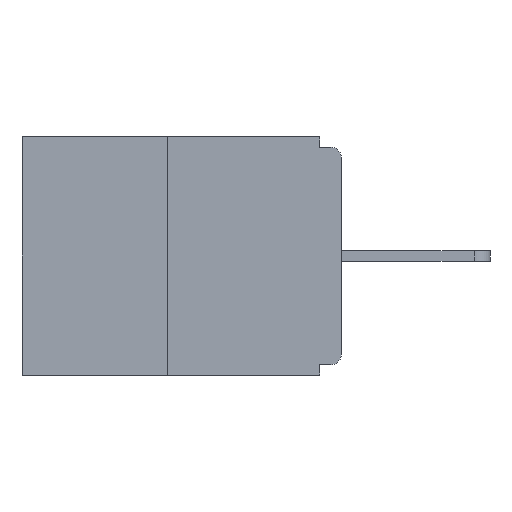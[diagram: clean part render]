
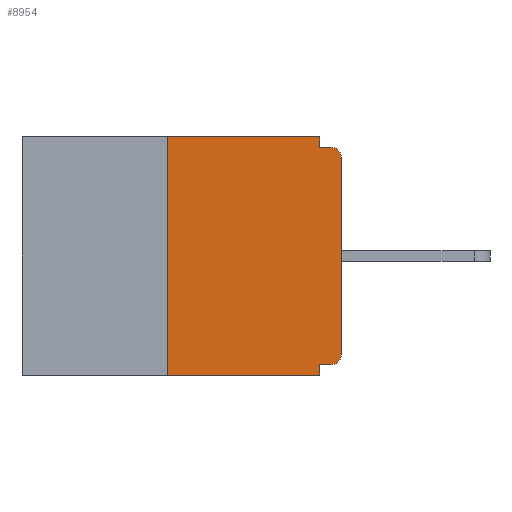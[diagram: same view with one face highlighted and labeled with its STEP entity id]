
A CAD part, left-side view. The second image highlights one B-rep face of the part: STEP entity #8954.
In plain terms, the highlighted planar face has unit normal (-1, 0, 0).
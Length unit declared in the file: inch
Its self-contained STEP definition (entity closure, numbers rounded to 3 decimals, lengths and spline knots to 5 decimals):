
#16 = CARTESIAN_POINT ( 'NONE',  ( 0., 0.015, -0.015 ) ) ;
#80 = VECTOR ( 'NONE', #10535, 39.37008 ) ;
#140 = ORIENTED_EDGE ( 'NONE', *, *, #8444, .F. ) ;
#161 = LINE ( 'NONE', #9205, #4442 ) ;
#212 = EDGE_CURVE ( 'NONE', #8233, #7573, #5155, .T. ) ;
#301 = VERTEX_POINT ( 'NONE', #8874 ) ;
#320 = ORIENTED_EDGE ( 'NONE', *, *, #418, .T. ) ;
#324 = CARTESIAN_POINT ( 'NONE',  ( 0., 0.46, 0. ) ) ;
#379 = DIRECTION ( 'NONE',  ( 0., 0., -1. ) ) ;
#418 = EDGE_CURVE ( 'NONE', #6286, #8233, #7456, .T. ) ;
#588 = DIRECTION ( 'NONE',  ( -1., 0., 0. ) ) ;
#603 = ORIENTED_EDGE ( 'NONE', *, *, #212, .T. ) ;
#849 = LINE ( 'NONE', #7314, #9579 ) ;
#899 = LINE ( 'NONE', #1636, #4601 ) ;
#989 = EDGE_CURVE ( 'NONE', #9513, #6377, #849, .T. ) ;
#1070 = FACE_OUTER_BOUND ( 'NONE', #1598, .T. ) ;
#1315 = VECTOR ( 'NONE', #6848, 39.37008 ) ;
#1461 = CARTESIAN_POINT ( 'NONE',  ( 0., 0., -0.328 ) ) ;
#1584 = CARTESIAN_POINT ( 'NONE',  ( 0., 0., -0.03 ) ) ;
#1594 = DIRECTION ( 'NONE',  ( 0., -1., 0. ) ) ;
#1598 = EDGE_LOOP ( 'NONE', ( #2621, #5974, #6229, #8746, #8062, #7811, #320, #603, #3981, #140 ) ) ;
#1636 = CARTESIAN_POINT ( 'NONE',  ( 0., 0.031, 0. ) ) ;
#1834 = LINE ( 'NONE', #324, #1315 ) ;
#2033 = AXIS2_PLACEMENT_3D ( 'NONE', #5449, #588, #6237 ) ;
#2140 = DIRECTION ( 'NONE',  ( 0., 0., -1. ) ) ;
#2203 = CARTESIAN_POINT ( 'NONE',  ( 0., 0.031, -0.343 ) ) ;
#2275 = LINE ( 'NONE', #1461, #5230 ) ;
#2278 = LINE ( 'NONE', #4780, #80 ) ;
#2409 = VERTEX_POINT ( 'NONE', #7207 ) ;
#2553 = CARTESIAN_POINT ( 'NONE',  ( 0., 0., 0. ) ) ;
#2621 = ORIENTED_EDGE ( 'NONE', *, *, #10112, .F. ) ;
#3011 = DIRECTION ( 'NONE',  ( -1., 0., 0. ) ) ;
#3078 = VERTEX_POINT ( 'NONE', #10090 ) ;
#3309 = CIRCLE ( 'NONE', #9323, 0.015 ) ;
#3534 = EDGE_CURVE ( 'NONE', #3078, #6286, #3309, .T. ) ;
#3981 = ORIENTED_EDGE ( 'NONE', *, *, #7483, .F. ) ;
#4133 = VECTOR ( 'NONE', #8020, 39.37008 ) ;
#4199 = DIRECTION ( 'NONE',  ( 0., 0., -1. ) ) ;
#4442 = VECTOR ( 'NONE', #5139, 39.37008 ) ;
#4601 = VECTOR ( 'NONE', #4199, 39.37008 ) ;
#4630 = EDGE_CURVE ( 'NONE', #3078, #9767, #2275, .T. ) ;
#4718 = CARTESIAN_POINT ( 'NONE',  ( 0., 0.031, -0.328 ) ) ;
#4780 = CARTESIAN_POINT ( 'NONE',  ( 0., 0., -0.015 ) ) ;
#5031 = PLANE ( 'NONE',  #5923 ) ;
#5133 = DIRECTION ( 'NONE',  ( 1., 0., 0. ) ) ;
#5139 = DIRECTION ( 'NONE',  ( 0., 0., 1. ) ) ;
#5155 = CIRCLE ( 'NONE', #2033, 0.015 ) ;
#5230 = VECTOR ( 'NONE', #7639, 39.37008 ) ;
#5240 = CARTESIAN_POINT ( 'NONE',  ( 0., 0., -0.313 ) ) ;
#5449 = CARTESIAN_POINT ( 'NONE',  ( 0., 0.015, -0.03 ) ) ;
#5496 = CARTESIAN_POINT ( 'NONE',  ( 0., 0.015, -0.313 ) ) ;
#5774 = CARTESIAN_POINT ( 'NONE',  ( 0., 0.46, 0. ) ) ;
#5923 = AXIS2_PLACEMENT_3D ( 'NONE', #5774, #5133, #10030 ) ;
#5929 = CARTESIAN_POINT ( 'NONE',  ( 0., 0.031, -0.343 ) ) ;
#5974 = ORIENTED_EDGE ( 'NONE', *, *, #10185, .F. ) ;
#6229 = ORIENTED_EDGE ( 'NONE', *, *, #989, .T. ) ;
#6237 = DIRECTION ( 'NONE',  ( 0., 0., -1. ) ) ;
#6286 = VERTEX_POINT ( 'NONE', #5240 ) ;
#6377 = VERTEX_POINT ( 'NONE', #5929 ) ;
#6848 = DIRECTION ( 'NONE',  ( 0., -1., 0. ) ) ;
#7207 = CARTESIAN_POINT ( 'NONE',  ( 0., 0.031, -0.015 ) ) ;
#7314 = CARTESIAN_POINT ( 'NONE',  ( 0., 0.46, -0.343 ) ) ;
#7449 = CARTESIAN_POINT ( 'NONE',  ( 0., 0.25, -0.343 ) ) ;
#7456 = LINE ( 'NONE', #2553, #4133 ) ;
#7483 = EDGE_CURVE ( 'NONE', #2409, #7573, #2278, .T. ) ;
#7573 = VERTEX_POINT ( 'NONE', #16 ) ;
#7639 = DIRECTION ( 'NONE',  ( 0., 1., 0. ) ) ;
#7811 = ORIENTED_EDGE ( 'NONE', *, *, #3534, .T. ) ;
#8016 = VECTOR ( 'NONE', #379, 39.37008 ) ;
#8020 = DIRECTION ( 'NONE',  ( 0., 0., 1. ) ) ;
#8062 = ORIENTED_EDGE ( 'NONE', *, *, #4630, .F. ) ;
#8233 = VERTEX_POINT ( 'NONE', #1584 ) ;
#8444 = EDGE_CURVE ( 'NONE', #9971, #2409, #899, .T. ) ;
#8561 = LINE ( 'NONE', #2203, #8016 ) ;
#8746 = ORIENTED_EDGE ( 'NONE', *, *, #10218, .F. ) ;
#8874 = CARTESIAN_POINT ( 'NONE',  ( 0., 0.25, 0. ) ) ;
#8954 = ADVANCED_FACE ( 'NONE', ( #1070 ), #5031, .F. ) ;
#9205 = CARTESIAN_POINT ( 'NONE',  ( 0., 0.25, 0. ) ) ;
#9323 = AXIS2_PLACEMENT_3D ( 'NONE', #5496, #3011, #2140 ) ;
#9513 = VERTEX_POINT ( 'NONE', #7449 ) ;
#9579 = VECTOR ( 'NONE', #1594, 39.37008 ) ;
#9767 = VERTEX_POINT ( 'NONE', #4718 ) ;
#9971 = VERTEX_POINT ( 'NONE', #10622 ) ;
#10030 = DIRECTION ( 'NONE',  ( 0., 0., -1. ) ) ;
#10090 = CARTESIAN_POINT ( 'NONE',  ( 0., 0.015, -0.328 ) ) ;
#10112 = EDGE_CURVE ( 'NONE', #301, #9971, #1834, .T. ) ;
#10185 = EDGE_CURVE ( 'NONE', #9513, #301, #161, .T. ) ;
#10218 = EDGE_CURVE ( 'NONE', #9767, #6377, #8561, .T. ) ;
#10535 = DIRECTION ( 'NONE',  ( 0., -1., 0. ) ) ;
#10622 = CARTESIAN_POINT ( 'NONE',  ( 0., 0.031, 0. ) ) ;
